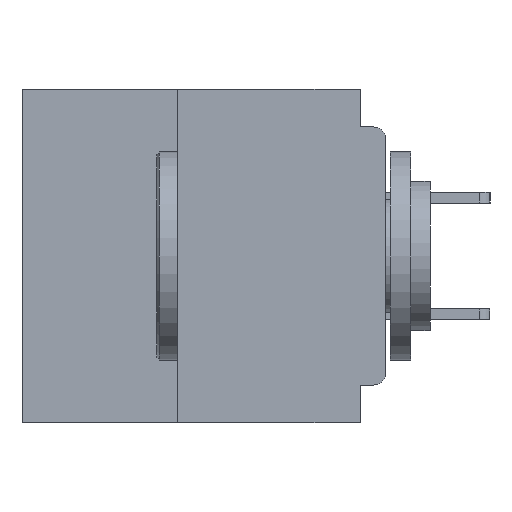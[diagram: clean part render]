
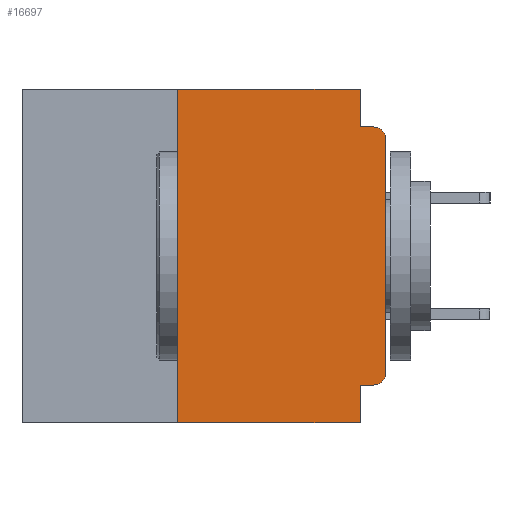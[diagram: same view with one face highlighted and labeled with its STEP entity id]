
A CAD part, left-side view. The second image highlights one B-rep face of the part: STEP entity #16697.
In plain terms, the highlighted planar face has unit normal (-1, 0, 0).
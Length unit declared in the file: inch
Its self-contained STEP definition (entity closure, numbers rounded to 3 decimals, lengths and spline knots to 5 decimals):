
#577 = CARTESIAN_POINT ( 'NONE',  ( 0., 0.015, -0.34 ) ) ;
#1286 = LINE ( 'NONE', #17232, #23327 ) ;
#2395 = ORIENTED_EDGE ( 'NONE', *, *, #23953, .T. ) ;
#2720 = DIRECTION ( 'NONE',  ( 0., 0., 1. ) ) ;
#3600 = DIRECTION ( 'NONE',  ( 0., 0., -1. ) ) ;
#3762 = AXIS2_PLACEMENT_3D ( 'NONE', #15820, #7245, #27216 ) ;
#3984 = CARTESIAN_POINT ( 'NONE',  ( 0., 0., -0.06 ) ) ;
#4331 = VERTEX_POINT ( 'NONE', #8715 ) ;
#4565 = CARTESIAN_POINT ( 'NONE',  ( 0., 0., 0. ) ) ;
#4834 = VERTEX_POINT ( 'NONE', #3984 ) ;
#5408 = VERTEX_POINT ( 'NONE', #23718 ) ;
#5982 = LINE ( 'NONE', #4565, #35209 ) ;
#7245 = DIRECTION ( 'NONE',  ( 1., 0., 0. ) ) ;
#7459 = DIRECTION ( 'NONE',  ( 0., 0., 1. ) ) ;
#7712 = ORIENTED_EDGE ( 'NONE', *, *, #24227, .F. ) ;
#7725 = CARTESIAN_POINT ( 'NONE',  ( 0., 0., -0.34 ) ) ;
#7948 = EDGE_CURVE ( 'NONE', #25490, #4834, #5982, .T. ) ;
#8490 = ORIENTED_EDGE ( 'NONE', *, *, #14356, .F. ) ;
#8715 = CARTESIAN_POINT ( 'NONE',  ( 0., 0.031, -0.4 ) ) ;
#9069 = FACE_OUTER_BOUND ( 'NONE', #25000, .T. ) ;
#9252 = ORIENTED_EDGE ( 'NONE', *, *, #35179, .F. ) ;
#10522 = CARTESIAN_POINT ( 'NONE',  ( 0., 0., -0.355 ) ) ;
#10952 = VERTEX_POINT ( 'NONE', #22239 ) ;
#11651 = CIRCLE ( 'NONE', #22466, 0.015 ) ;
#11833 = CARTESIAN_POINT ( 'NONE',  ( 0., 0.015, -0.06 ) ) ;
#11910 = VECTOR ( 'NONE', #14549, 39.37008 ) ;
#14038 = EDGE_CURVE ( 'NONE', #5408, #24005, #22668, .T. ) ;
#14250 = EDGE_CURVE ( 'NONE', #10952, #4331, #30649, .T. ) ;
#14356 = EDGE_CURVE ( 'NONE', #24005, #30508, #19589, .T. ) ;
#14549 = DIRECTION ( 'NONE',  ( 0., 0., -1. ) ) ;
#14756 = DIRECTION ( 'NONE',  ( 0., 0., -1. ) ) ;
#15123 = VECTOR ( 'NONE', #35085, 39.37008 ) ;
#15319 = CARTESIAN_POINT ( 'NONE',  ( 0., 0.031, 0. ) ) ;
#15820 = CARTESIAN_POINT ( 'NONE',  ( 0., 0.437, 0. ) ) ;
#16005 = ORIENTED_EDGE ( 'NONE', *, *, #27647, .F. ) ;
#16697 = ADVANCED_FACE ( 'NONE', ( #9069 ), #18588, .F. ) ;
#16845 = DIRECTION ( 'NONE',  ( 0., -1., 0. ) ) ;
#16911 = ORIENTED_EDGE ( 'NONE', *, *, #14250, .T. ) ;
#17232 = CARTESIAN_POINT ( 'NONE',  ( 0., 0., -0.045 ) ) ;
#17529 = CARTESIAN_POINT ( 'NONE',  ( 0., 0.031, -0.4 ) ) ;
#18588 = PLANE ( 'NONE',  #3762 ) ;
#19070 = ORIENTED_EDGE ( 'NONE', *, *, #35911, .T. ) ;
#19184 = VECTOR ( 'NONE', #20359, 39.37008 ) ;
#19589 = LINE ( 'NONE', #34120, #11910 ) ;
#19852 = VERTEX_POINT ( 'NONE', #35283 ) ;
#20100 = CARTESIAN_POINT ( 'NONE',  ( 0., 0.015, -0.355 ) ) ;
#20359 = DIRECTION ( 'NONE',  ( 0., 0., -1. ) ) ;
#20798 = DIRECTION ( 'NONE',  ( -1., 0., 0. ) ) ;
#21205 = AXIS2_PLACEMENT_3D ( 'NONE', #577, #20798, #3600 ) ;
#22239 = CARTESIAN_POINT ( 'NONE',  ( 0., 0.25, -0.4 ) ) ;
#22466 = AXIS2_PLACEMENT_3D ( 'NONE', #11833, #31731, #14756 ) ;
#22650 = ORIENTED_EDGE ( 'NONE', *, *, #14038, .F. ) ;
#22668 = LINE ( 'NONE', #32387, #15123 ) ;
#23089 = VECTOR ( 'NONE', #16845, 39.37008 ) ;
#23327 = VECTOR ( 'NONE', #36716, 39.37008 ) ;
#23399 = LINE ( 'NONE', #10522, #30088 ) ;
#23718 = CARTESIAN_POINT ( 'NONE',  ( 0., 0.25, 0. ) ) ;
#23953 = EDGE_CURVE ( 'NONE', #28457, #25490, #25157, .T. ) ;
#24005 = VERTEX_POINT ( 'NONE', #15319 ) ;
#24227 = EDGE_CURVE ( 'NONE', #28457, #29549, #23399, .T. ) ;
#24894 = ORIENTED_EDGE ( 'NONE', *, *, #7948, .T. ) ;
#25000 = EDGE_LOOP ( 'NONE', ( #24894, #19070, #9252, #8490, #22650, #25788, #16911, #16005, #7712, #2395 ) ) ;
#25157 = CIRCLE ( 'NONE', #21205, 0.015 ) ;
#25490 = VERTEX_POINT ( 'NONE', #7725 ) ;
#25788 = ORIENTED_EDGE ( 'NONE', *, *, #26353, .F. ) ;
#25902 = VECTOR ( 'NONE', #2720, 39.37008 ) ;
#26353 = EDGE_CURVE ( 'NONE', #10952, #5408, #33307, .T. ) ;
#27216 = DIRECTION ( 'NONE',  ( 0., 0., -1. ) ) ;
#27647 = EDGE_CURVE ( 'NONE', #29549, #4331, #34051, .T. ) ;
#28457 = VERTEX_POINT ( 'NONE', #20100 ) ;
#29549 = VERTEX_POINT ( 'NONE', #35865 ) ;
#30088 = VECTOR ( 'NONE', #30450, 39.37008 ) ;
#30450 = DIRECTION ( 'NONE',  ( 0., 1., 0. ) ) ;
#30508 = VERTEX_POINT ( 'NONE', #34384 ) ;
#30649 = LINE ( 'NONE', #36360, #23089 ) ;
#31731 = DIRECTION ( 'NONE',  ( -1., 0., 0. ) ) ;
#32387 = CARTESIAN_POINT ( 'NONE',  ( 0., 0.437, 0. ) ) ;
#33307 = LINE ( 'NONE', #34149, #25902 ) ;
#34051 = LINE ( 'NONE', #17529, #19184 ) ;
#34120 = CARTESIAN_POINT ( 'NONE',  ( 0., 0.031, 0. ) ) ;
#34149 = CARTESIAN_POINT ( 'NONE',  ( 0., 0.25, -0.4 ) ) ;
#34384 = CARTESIAN_POINT ( 'NONE',  ( 0., 0.031, -0.045 ) ) ;
#35085 = DIRECTION ( 'NONE',  ( 0., -1., 0. ) ) ;
#35179 = EDGE_CURVE ( 'NONE', #30508, #19852, #1286, .T. ) ;
#35209 = VECTOR ( 'NONE', #7459, 39.37008 ) ;
#35283 = CARTESIAN_POINT ( 'NONE',  ( 0., 0.015, -0.045 ) ) ;
#35865 = CARTESIAN_POINT ( 'NONE',  ( 0., 0.031, -0.355 ) ) ;
#35911 = EDGE_CURVE ( 'NONE', #4834, #19852, #11651, .T. ) ;
#36360 = CARTESIAN_POINT ( 'NONE',  ( 0., 0.437, -0.4 ) ) ;
#36716 = DIRECTION ( 'NONE',  ( 0., -1., 0. ) ) ;
